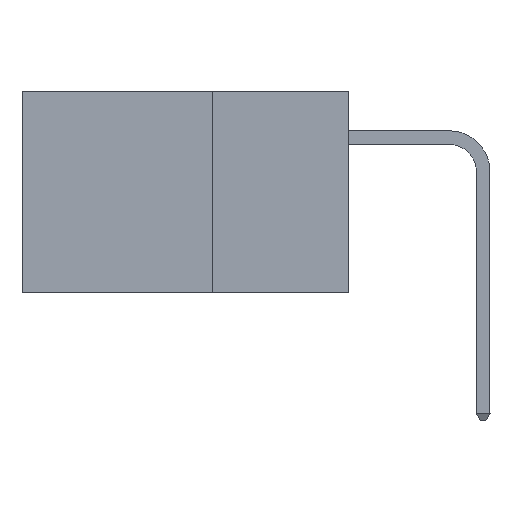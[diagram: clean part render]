
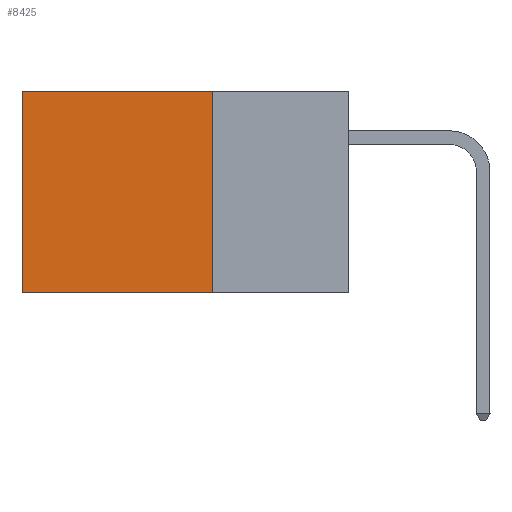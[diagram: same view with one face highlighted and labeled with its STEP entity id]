
A CAD part, left-side view. The second image highlights one B-rep face of the part: STEP entity #8425.
In plain terms, the highlighted planar face has unit normal (-1, 0, 0).
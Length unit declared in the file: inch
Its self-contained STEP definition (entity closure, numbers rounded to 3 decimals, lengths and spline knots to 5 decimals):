
#605 = CARTESIAN_POINT ( 'NONE',  ( 0.2875, 0.6, 0. ) ) ;
#1123 = EDGE_CURVE ( 'NONE', #10564, #11935, #3282, .T. ) ;
#3282 = LINE ( 'NONE', #9091, #24000 ) ;
#3361 = CARTESIAN_POINT ( 'NONE',  ( 0.2875, 0.25, -0.37 ) ) ;
#3672 = LINE ( 'NONE', #13255, #33935 ) ;
#4265 = DIRECTION ( 'NONE',  ( 0., 1., 0. ) ) ;
#5128 = EDGE_LOOP ( 'NONE', ( #38115, #13621, #22661, #15120 ) ) ;
#8275 = EDGE_CURVE ( 'NONE', #10564, #26703, #30711, .T. ) ;
#8425 = ADVANCED_FACE ( 'NONE', ( #16512 ), #22300, .F. ) ;
#9091 = CARTESIAN_POINT ( 'NONE',  ( 0.2875, 0.25, 0. ) ) ;
#9727 = CARTESIAN_POINT ( 'NONE',  ( 0.2875, 0.25, 0. ) ) ;
#10322 = DIRECTION ( 'NONE',  ( 1., 0., 0. ) ) ;
#10564 = VERTEX_POINT ( 'NONE', #27238 ) ;
#11135 = VECTOR ( 'NONE', #34010, 39.37008 ) ;
#11935 = VERTEX_POINT ( 'NONE', #3361 ) ;
#12121 = DIRECTION ( 'NONE',  ( 0., 1., 0. ) ) ;
#13255 = CARTESIAN_POINT ( 'NONE',  ( 0.2875, 0.25, -0.37 ) ) ;
#13621 = ORIENTED_EDGE ( 'NONE', *, *, #35263, .F. ) ;
#14181 = VERTEX_POINT ( 'NONE', #25839 ) ;
#14461 = EDGE_CURVE ( 'NONE', #26703, #14181, #15621, .T. ) ;
#15120 = ORIENTED_EDGE ( 'NONE', *, *, #8275, .T. ) ;
#15322 = CARTESIAN_POINT ( 'NONE',  ( 0.2875, 0.25, 0. ) ) ;
#15621 = LINE ( 'NONE', #605, #11135 ) ;
#15722 = DIRECTION ( 'NONE',  ( 0., 0., -1. ) ) ;
#16512 = FACE_OUTER_BOUND ( 'NONE', #5128, .T. ) ;
#21871 = DIRECTION ( 'NONE',  ( 0., 0., -1. ) ) ;
#22300 = PLANE ( 'NONE',  #26165 ) ;
#22661 = ORIENTED_EDGE ( 'NONE', *, *, #1123, .F. ) ;
#24000 = VECTOR ( 'NONE', #21871, 39.37008 ) ;
#25839 = CARTESIAN_POINT ( 'NONE',  ( 0.2875, 0.6, -0.37 ) ) ;
#26165 = AXIS2_PLACEMENT_3D ( 'NONE', #9727, #10322, #15722 ) ;
#26703 = VERTEX_POINT ( 'NONE', #35377 ) ;
#27238 = CARTESIAN_POINT ( 'NONE',  ( 0.2875, 0.25, 0. ) ) ;
#28734 = VECTOR ( 'NONE', #12121, 39.37008 ) ;
#30711 = LINE ( 'NONE', #15322, #28734 ) ;
#33935 = VECTOR ( 'NONE', #4265, 39.37008 ) ;
#34010 = DIRECTION ( 'NONE',  ( 0., 0., -1. ) ) ;
#35263 = EDGE_CURVE ( 'NONE', #11935, #14181, #3672, .T. ) ;
#35377 = CARTESIAN_POINT ( 'NONE',  ( 0.2875, 0.6, 0. ) ) ;
#38115 = ORIENTED_EDGE ( 'NONE', *, *, #14461, .T. ) ;
